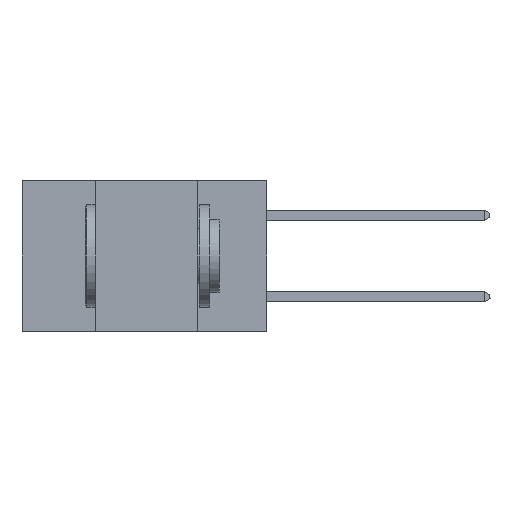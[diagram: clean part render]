
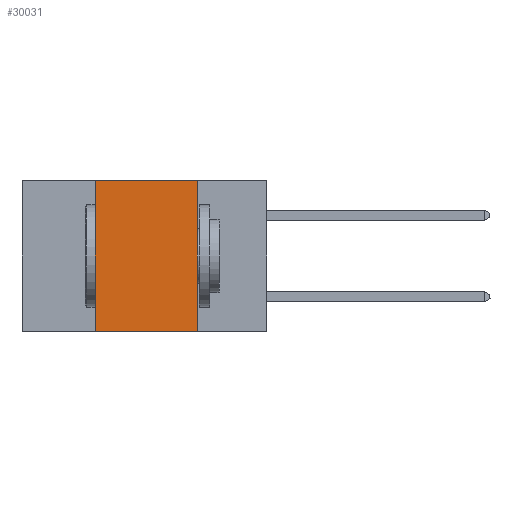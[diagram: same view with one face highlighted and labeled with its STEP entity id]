
A CAD part, left-side view. The second image highlights one B-rep face of the part: STEP entity #30031.
In plain terms, the highlighted planar face has unit normal (-1, 0, 0).
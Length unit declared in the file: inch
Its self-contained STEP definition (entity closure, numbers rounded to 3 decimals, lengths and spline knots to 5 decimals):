
#574 = LINE ( 'NONE', #9259, #36146 ) ;
#1405 = VERTEX_POINT ( 'NONE', #2243 ) ;
#2243 = CARTESIAN_POINT ( 'NONE',  ( 0., 0.42, -0.37 ) ) ;
#2873 = CARTESIAN_POINT ( 'NONE',  ( 0., 0.17, 0. ) ) ;
#3727 = VERTEX_POINT ( 'NONE', #9868 ) ;
#4238 = CARTESIAN_POINT ( 'NONE',  ( 0., 0.42, 0. ) ) ;
#8856 = DIRECTION ( 'NONE',  ( 1., 0., 0. ) ) ;
#9259 = CARTESIAN_POINT ( 'NONE',  ( 0., 0.6, 0. ) ) ;
#9868 = CARTESIAN_POINT ( 'NONE',  ( 0., 0.17, 0. ) ) ;
#9869 = FACE_OUTER_BOUND ( 'NONE', #23247, .T. ) ;
#12182 = VECTOR ( 'NONE', #25762, 39.37008 ) ;
#14868 = VECTOR ( 'NONE', #36315, 39.37008 ) ;
#15735 = DIRECTION ( 'NONE',  ( 0., 0., 1. ) ) ;
#16653 = ORIENTED_EDGE ( 'NONE', *, *, #36352, .T. ) ;
#20428 = VERTEX_POINT ( 'NONE', #31225 ) ;
#21220 = ORIENTED_EDGE ( 'NONE', *, *, #32427, .F. ) ;
#23247 = EDGE_LOOP ( 'NONE', ( #33409, #27739, #21220, #16653 ) ) ;
#23918 = CARTESIAN_POINT ( 'NONE',  ( 0., 0.17, -0.37 ) ) ;
#23951 = EDGE_CURVE ( 'NONE', #3727, #32354, #36780, .T. ) ;
#25762 = DIRECTION ( 'NONE',  ( 0., 0., -1. ) ) ;
#26151 = VECTOR ( 'NONE', #15735, 39.37008 ) ;
#27739 = ORIENTED_EDGE ( 'NONE', *, *, #37342, .F. ) ;
#29777 = LINE ( 'NONE', #4238, #26151 ) ;
#30031 = ADVANCED_FACE ( 'NONE', ( #9869 ), #31927, .F. ) ;
#31225 = CARTESIAN_POINT ( 'NONE',  ( 0., 0.42, 0. ) ) ;
#31927 = PLANE ( 'NONE',  #37489 ) ;
#32354 = VERTEX_POINT ( 'NONE', #23918 ) ;
#32427 = EDGE_CURVE ( 'NONE', #1405, #20428, #29777, .T. ) ;
#33409 = ORIENTED_EDGE ( 'NONE', *, *, #23951, .F. ) ;
#33677 = CARTESIAN_POINT ( 'NONE',  ( 0., 0.6, -0.37 ) ) ;
#33978 = LINE ( 'NONE', #33677, #14868 ) ;
#34817 = DIRECTION ( 'NONE',  ( 0., 0., -1. ) ) ;
#35281 = CARTESIAN_POINT ( 'NONE',  ( 0., 0.6, 0. ) ) ;
#35849 = DIRECTION ( 'NONE',  ( 0., -1., 0. ) ) ;
#36146 = VECTOR ( 'NONE', #35849, 39.37008 ) ;
#36315 = DIRECTION ( 'NONE',  ( 0., -1., 0. ) ) ;
#36352 = EDGE_CURVE ( 'NONE', #1405, #32354, #33978, .T. ) ;
#36780 = LINE ( 'NONE', #2873, #12182 ) ;
#37342 = EDGE_CURVE ( 'NONE', #20428, #3727, #574, .T. ) ;
#37489 = AXIS2_PLACEMENT_3D ( 'NONE', #35281, #8856, #34817 ) ;
